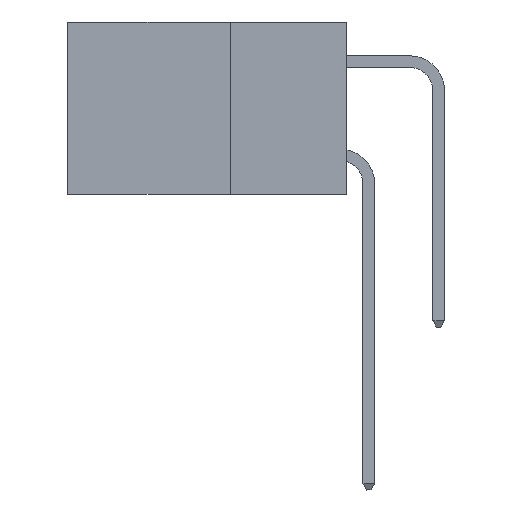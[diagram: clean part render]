
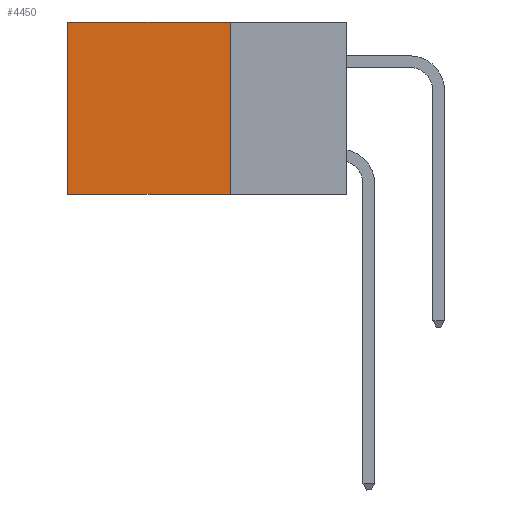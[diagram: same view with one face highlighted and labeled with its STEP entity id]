
A CAD part, left-side view. The second image highlights one B-rep face of the part: STEP entity #4450.
In plain terms, the highlighted planar face has unit normal (-1, 0, 0).
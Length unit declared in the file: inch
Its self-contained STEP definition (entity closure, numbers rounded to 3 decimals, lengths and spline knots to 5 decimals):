
#599 = VECTOR ( 'NONE', #11715, 39.37008 ) ;
#633 = CARTESIAN_POINT ( 'NONE',  ( 0.2875, 0.25, -0.37 ) ) ;
#1319 = CARTESIAN_POINT ( 'NONE',  ( 0.2875, 0.6, -0.37 ) ) ;
#1395 = ORIENTED_EDGE ( 'NONE', *, *, #4124, .T. ) ;
#3382 = EDGE_CURVE ( 'NONE', #12151, #21194, #20353, .T. ) ;
#4124 = EDGE_CURVE ( 'NONE', #20868, #10361, #10972, .T. ) ;
#4450 = ADVANCED_FACE ( 'NONE', ( #15504 ), #9546, .F. ) ;
#4478 = CARTESIAN_POINT ( 'NONE',  ( 0.2875, 0.6, 0. ) ) ;
#4854 = EDGE_CURVE ( 'NONE', #21194, #10361, #14867, .T. ) ;
#5984 = DIRECTION ( 'NONE',  ( 1., 0., 0. ) ) ;
#6266 = ORIENTED_EDGE ( 'NONE', *, *, #3382, .F. ) ;
#7144 = AXIS2_PLACEMENT_3D ( 'NONE', #22208, #5984, #11352 ) ;
#8806 = ORIENTED_EDGE ( 'NONE', *, *, #4854, .F. ) ;
#9523 = DIRECTION ( 'NONE',  ( 0., 1., 0. ) ) ;
#9546 = PLANE ( 'NONE',  #7144 ) ;
#10361 = VERTEX_POINT ( 'NONE', #1319 ) ;
#10787 = CARTESIAN_POINT ( 'NONE',  ( 0.2875, 0.25, 0. ) ) ;
#10972 = LINE ( 'NONE', #4478, #17796 ) ;
#11352 = DIRECTION ( 'NONE',  ( 0., 0., -1. ) ) ;
#11644 = LINE ( 'NONE', #18946, #599 ) ;
#11715 = DIRECTION ( 'NONE',  ( 0., 1., 0. ) ) ;
#12151 = VERTEX_POINT ( 'NONE', #20141 ) ;
#12287 = CARTESIAN_POINT ( 'NONE',  ( 0.2875, 0.25, -0.37 ) ) ;
#13479 = VECTOR ( 'NONE', #9523, 39.37008 ) ;
#14867 = LINE ( 'NONE', #633, #13479 ) ;
#15504 = FACE_OUTER_BOUND ( 'NONE', #18276, .T. ) ;
#16675 = VECTOR ( 'NONE', #23128, 39.37008 ) ;
#17796 = VECTOR ( 'NONE', #20426, 39.37008 ) ;
#18276 = EDGE_LOOP ( 'NONE', ( #1395, #8806, #6266, #22649 ) ) ;
#18946 = CARTESIAN_POINT ( 'NONE',  ( 0.2875, 0.25, 0. ) ) ;
#20141 = CARTESIAN_POINT ( 'NONE',  ( 0.2875, 0.25, 0. ) ) ;
#20353 = LINE ( 'NONE', #10787, #16675 ) ;
#20426 = DIRECTION ( 'NONE',  ( 0., 0., -1. ) ) ;
#20868 = VERTEX_POINT ( 'NONE', #22678 ) ;
#21194 = VERTEX_POINT ( 'NONE', #12287 ) ;
#21533 = EDGE_CURVE ( 'NONE', #12151, #20868, #11644, .T. ) ;
#22208 = CARTESIAN_POINT ( 'NONE',  ( 0.2875, 0.25, 0. ) ) ;
#22649 = ORIENTED_EDGE ( 'NONE', *, *, #21533, .T. ) ;
#22678 = CARTESIAN_POINT ( 'NONE',  ( 0.2875, 0.6, 0. ) ) ;
#23128 = DIRECTION ( 'NONE',  ( 0., 0., -1. ) ) ;
